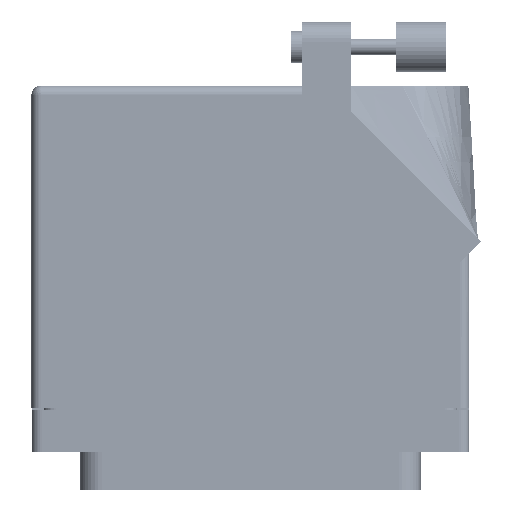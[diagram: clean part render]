
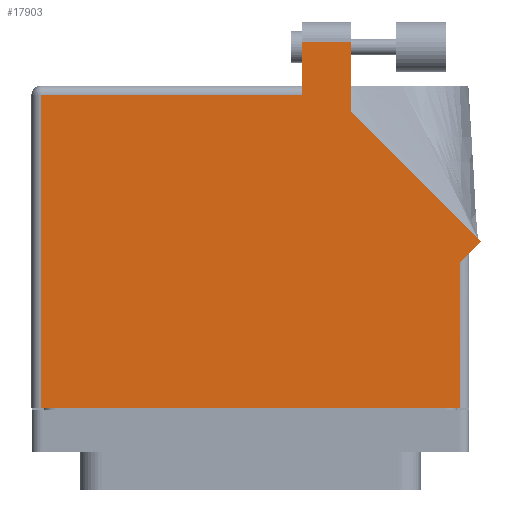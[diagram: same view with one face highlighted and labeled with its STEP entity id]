
A CAD part, front view. The second image highlights one B-rep face of the part: STEP entity #17903.
In plain terms, the highlighted face is planar.
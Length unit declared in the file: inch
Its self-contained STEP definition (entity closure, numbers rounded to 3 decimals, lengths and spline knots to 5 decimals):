
#5646 = LINE ( 'NONE', #13532, #85214 ) ;
#7168 = DIRECTION ( 'NONE',  ( 0.707, 0.707, 0. ) ) ;
#7561 = AXIS2_PLACEMENT_3D ( 'NONE', #64371, #71258, #28088 ) ;
#8728 = EDGE_LOOP ( 'NONE', ( #80079, #75432, #37287, #52034, #54670, #81151, #85213, #67385, #79091 ) ) ;
#8970 = LINE ( 'NONE', #29407, #41537 ) ;
#9150 = VECTOR ( 'NONE', #72395, 39.37008 ) ;
#10456 = EDGE_CURVE ( 'NONE', #56450, #19370, #8970, .T. ) ;
#11304 = EDGE_CURVE ( 'NONE', #58198, #70299, #28927, .T. ) ;
#13532 = CARTESIAN_POINT ( 'NONE',  ( 0.6345, 1.76442, 0.765 ) ) ;
#13664 = CARTESIAN_POINT ( 'NONE',  ( 1.44821, 0.95071, 0.765 ) ) ;
#13982 = DIRECTION ( 'NONE',  ( 0., -1., 0. ) ) ;
#16210 = CARTESIAN_POINT ( 'NONE',  ( 0.3275, 2.205, 0.765 ) ) ;
#17268 = VECTOR ( 'NONE', #47642, 39.37008 ) ;
#17903 = ADVANCED_FACE ( 'NONE', ( #46981 ), #85940, .F. ) ;
#18265 = LINE ( 'NONE', #22469, #55169 ) ;
#19370 = VERTEX_POINT ( 'NONE', #81018 ) ;
#22223 = VERTEX_POINT ( 'NONE', #16210 ) ;
#22469 = CARTESIAN_POINT ( 'NONE',  ( 0.3275, 2.205, 0.765 ) ) ;
#23615 = DIRECTION ( 'NONE',  ( 0., -1., 0. ) ) ;
#28088 = DIRECTION ( 'NONE',  ( -1., 0., 0. ) ) ;
#28110 = LINE ( 'NONE', #13664, #72887 ) ;
#28154 = VERTEX_POINT ( 'NONE', #88950 ) ;
#28181 = CARTESIAN_POINT ( 'NONE',  ( 0.6345, 1.76442, 0.765 ) ) ;
#28199 = VERTEX_POINT ( 'NONE', #61096 ) ;
#28289 = LINE ( 'NONE', #64606, #9150 ) ;
#28927 = LINE ( 'NONE', #71750, #49132 ) ;
#29407 = CARTESIAN_POINT ( 'NONE',  ( -1.3775, -0.1, 0.765 ) ) ;
#29629 = DIRECTION ( 'NONE',  ( -1., 0., 0. ) ) ;
#34619 = CARTESIAN_POINT ( 'NONE',  ( -1.3155, -0.1, 0.765 ) ) ;
#36296 = LINE ( 'NONE', #56023, #17268 ) ;
#37287 = ORIENTED_EDGE ( 'NONE', *, *, #43560, .T. ) ;
#39490 = VECTOR ( 'NONE', #13982, 39.37008 ) ;
#40531 = CARTESIAN_POINT ( 'NONE',  ( 1.44821, 0.95071, 0.765 ) ) ;
#40641 = CARTESIAN_POINT ( 'NONE',  ( 1.3155, 0.818, 0.765 ) ) ;
#41537 = VECTOR ( 'NONE', #57868, 39.37008 ) ;
#41940 = CARTESIAN_POINT ( 'NONE',  ( 0.3275, 1.868, 0.765 ) ) ;
#43560 = EDGE_CURVE ( 'NONE', #22223, #51518, #63282, .T. ) ;
#45329 = EDGE_CURVE ( 'NONE', #19370, #58198, #28289, .T. ) ;
#46981 = FACE_OUTER_BOUND ( 'NONE', #8728, .T. ) ;
#47642 = DIRECTION ( 'NONE',  ( -1., 0., 0. ) ) ;
#49132 = VECTOR ( 'NONE', #7168, 39.37008 ) ;
#50361 = CARTESIAN_POINT ( 'NONE',  ( -1.3155, -0.1, 0.765 ) ) ;
#51518 = VERTEX_POINT ( 'NONE', #41940 ) ;
#52034 = ORIENTED_EDGE ( 'NONE', *, *, #71917, .T. ) ;
#54670 = ORIENTED_EDGE ( 'NONE', *, *, #78755, .T. ) ;
#55169 = VECTOR ( 'NONE', #29629, 39.37008 ) ;
#56023 = CARTESIAN_POINT ( 'NONE',  ( -1.3775, 1.868, 0.765 ) ) ;
#56450 = VERTEX_POINT ( 'NONE', #34619 ) ;
#57056 = EDGE_CURVE ( 'NONE', #82817, #28199, #5646, .T. ) ;
#57690 = VECTOR ( 'NONE', #23615, 39.37008 ) ;
#57868 = DIRECTION ( 'NONE',  ( 1., 0., 0. ) ) ;
#58198 = VERTEX_POINT ( 'NONE', #40641 ) ;
#61096 = CARTESIAN_POINT ( 'NONE',  ( 0.6345, 2.205, 0.765 ) ) ;
#63004 = LINE ( 'NONE', #50361, #39490 ) ;
#63020 = EDGE_CURVE ( 'NONE', #70299, #82817, #28110, .T. ) ;
#63282 = LINE ( 'NONE', #73966, #57690 ) ;
#64371 = CARTESIAN_POINT ( 'NONE',  ( -1.3775, 1.93, 0.765 ) ) ;
#64606 = CARTESIAN_POINT ( 'NONE',  ( 1.3155, 0.88, 0.765 ) ) ;
#67385 = ORIENTED_EDGE ( 'NONE', *, *, #11304, .T. ) ;
#70227 = DIRECTION ( 'NONE',  ( 0., 1., 0. ) ) ;
#70299 = VERTEX_POINT ( 'NONE', #40531 ) ;
#70986 = DIRECTION ( 'NONE',  ( -0.707, 0.707, 0. ) ) ;
#71258 = DIRECTION ( 'NONE',  ( 0., 0., -1. ) ) ;
#71750 = CARTESIAN_POINT ( 'NONE',  ( 1.3775, 0.88, 0.765 ) ) ;
#71917 = EDGE_CURVE ( 'NONE', #51518, #28154, #36296, .T. ) ;
#72395 = DIRECTION ( 'NONE',  ( 0., 1., 0. ) ) ;
#72599 = EDGE_CURVE ( 'NONE', #28199, #22223, #18265, .T. ) ;
#72887 = VECTOR ( 'NONE', #70986, 39.37008 ) ;
#73966 = CARTESIAN_POINT ( 'NONE',  ( 0.3275, 1.93, 0.765 ) ) ;
#75432 = ORIENTED_EDGE ( 'NONE', *, *, #72599, .T. ) ;
#78755 = EDGE_CURVE ( 'NONE', #28154, #56450, #63004, .T. ) ;
#79091 = ORIENTED_EDGE ( 'NONE', *, *, #63020, .T. ) ;
#80079 = ORIENTED_EDGE ( 'NONE', *, *, #57056, .T. ) ;
#81018 = CARTESIAN_POINT ( 'NONE',  ( 1.3155, -0.1, 0.765 ) ) ;
#81151 = ORIENTED_EDGE ( 'NONE', *, *, #10456, .T. ) ;
#82817 = VERTEX_POINT ( 'NONE', #28181 ) ;
#85213 = ORIENTED_EDGE ( 'NONE', *, *, #45329, .T. ) ;
#85214 = VECTOR ( 'NONE', #70227, 39.37008 ) ;
#85940 = PLANE ( 'NONE',  #7561 ) ;
#88950 = CARTESIAN_POINT ( 'NONE',  ( -1.3155, 1.868, 0.765 ) ) ;
